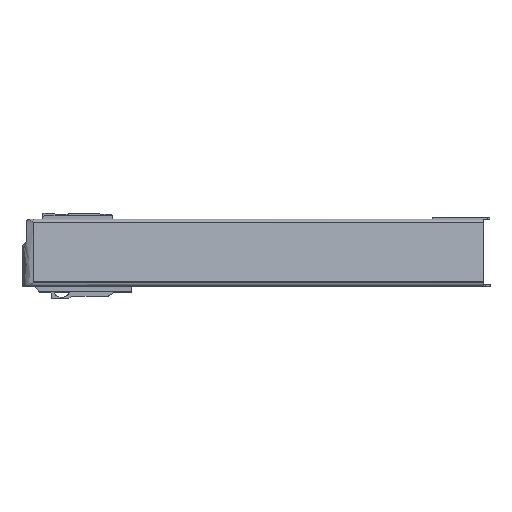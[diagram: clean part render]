
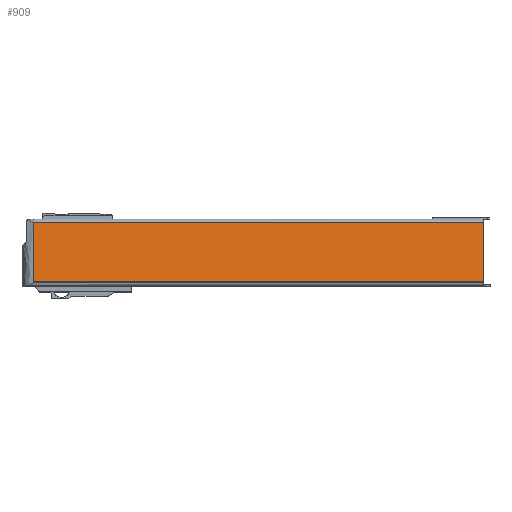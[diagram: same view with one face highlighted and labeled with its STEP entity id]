
A CAD part, top view. The second image highlights one B-rep face of the part: STEP entity #909.
In plain terms, the highlighted planar face has unit normal (0, 0.106, 0.994).
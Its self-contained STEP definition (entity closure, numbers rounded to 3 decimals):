
#245 = EDGE_CURVE ( 'NONE', #5672, #7621, #3716, .T. ) ;
#452 = DIRECTION ( 'NONE',  ( -1., 0., 0. ) ) ;
#507 = ORIENTED_EDGE ( 'NONE', *, *, #4604, .T. ) ;
#793 = CARTESIAN_POINT ( 'NONE',  ( 0., 0., 12.5 ) ) ;
#909 = ADVANCED_FACE ( 'NONE', ( #5027 ), #7551, .F. ) ;
#1180 = ORIENTED_EDGE ( 'NONE', *, *, #6240, .F. ) ;
#1217 = DIRECTION ( 'NONE',  ( 0., -0.994, 0.106 ) ) ;
#1482 = VERTEX_POINT ( 'NONE', #2523 ) ;
#2523 = CARTESIAN_POINT ( 'NONE',  ( 220., 31.112, 9.19 ) ) ;
#2567 = VECTOR ( 'NONE', #452, 1000. ) ;
#2846 = CARTESIAN_POINT ( 'NONE',  ( 220., 31.112, 9.19 ) ) ;
#2885 = LINE ( 'NONE', #2846, #2567 ) ;
#2919 = CARTESIAN_POINT ( 'NONE',  ( 0., 2.212, 12.265 ) ) ;
#3222 = DIRECTION ( 'NONE',  ( 1., 0., 0. ) ) ;
#3496 = EDGE_CURVE ( 'NONE', #1482, #7001, #2885, .T. ) ;
#3716 = LINE ( 'NONE', #7480, #5852 ) ;
#3889 = CARTESIAN_POINT ( 'NONE',  ( 0., 31.112, 9.19 ) ) ;
#3964 = LINE ( 'NONE', #4347, #5874 ) ;
#4012 = AXIS2_PLACEMENT_3D ( 'NONE', #4402, #6932, #5683 ) ;
#4347 = CARTESIAN_POINT ( 'NONE',  ( 220., 0., 12.5 ) ) ;
#4402 = CARTESIAN_POINT ( 'NONE',  ( 220., 0., 12.5 ) ) ;
#4580 = LINE ( 'NONE', #793, #7189 ) ;
#4604 = EDGE_CURVE ( 'NONE', #7001, #5672, #4580, .T. ) ;
#5027 = FACE_OUTER_BOUND ( 'NONE', #7337, .T. ) ;
#5091 = ORIENTED_EDGE ( 'NONE', *, *, #245, .T. ) ;
#5672 = VERTEX_POINT ( 'NONE', #2919 ) ;
#5683 = DIRECTION ( 'NONE',  ( 0., 0.994, -0.106 ) ) ;
#5852 = VECTOR ( 'NONE', #3222, 1000. ) ;
#5874 = VECTOR ( 'NONE', #1217, 1000. ) ;
#6240 = EDGE_CURVE ( 'NONE', #1482, #7621, #3964, .T. ) ;
#6649 = ORIENTED_EDGE ( 'NONE', *, *, #3496, .T. ) ;
#6932 = DIRECTION ( 'NONE',  ( 0., -0.106, -0.994 ) ) ;
#7001 = VERTEX_POINT ( 'NONE', #3889 ) ;
#7079 = CARTESIAN_POINT ( 'NONE',  ( 220., 2.212, 12.265 ) ) ;
#7178 = DIRECTION ( 'NONE',  ( 0., -0.994, 0.106 ) ) ;
#7189 = VECTOR ( 'NONE', #7178, 1000. ) ;
#7337 = EDGE_LOOP ( 'NONE', ( #507, #5091, #1180, #6649 ) ) ;
#7480 = CARTESIAN_POINT ( 'NONE',  ( 220., 2.212, 12.265 ) ) ;
#7551 = PLANE ( 'NONE',  #4012 ) ;
#7621 = VERTEX_POINT ( 'NONE', #7079 ) ;
